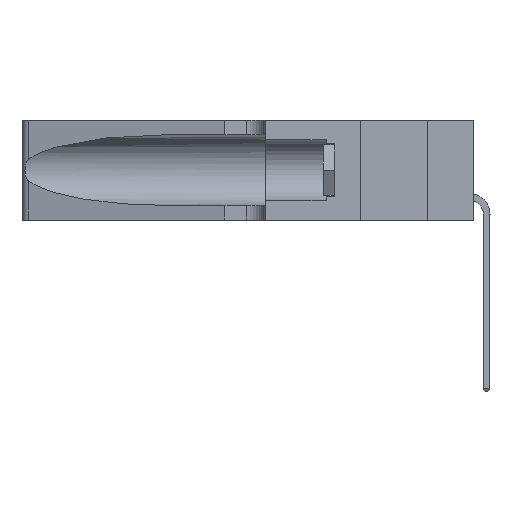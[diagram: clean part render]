
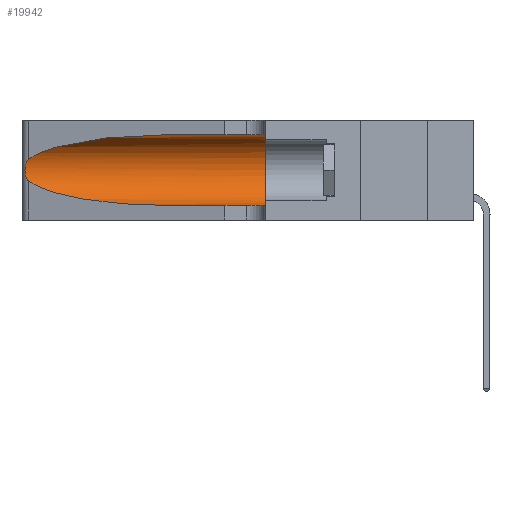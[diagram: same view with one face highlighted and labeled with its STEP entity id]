
A CAD part, left-side view. The second image highlights one B-rep face of the part: STEP entity #19942.
In plain terms, the highlighted cylindrical face has radius 3.308 mm (diameter 6.617 mm), a partial arc.
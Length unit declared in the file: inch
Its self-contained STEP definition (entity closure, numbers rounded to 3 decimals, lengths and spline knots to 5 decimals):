
#207 = ORIENTED_EDGE ( 'NONE', *, *, #4473, .T. ) ;
#224 = CYLINDRICAL_SURFACE ( 'NONE', #10447, 0.13025 ) ;
#479 = CARTESIAN_POINT ( 'NONE',  ( 0.1305, 0.35, 0.185 ) ) ;
#815 = VERTEX_POINT ( 'NONE', #22524 ) ;
#1253 = VERTEX_POINT ( 'NONE', #10271 ) ;
#1884 = ORIENTED_EDGE ( 'NONE', *, *, #13714, .T. ) ;
#2451 = EDGE_CURVE ( 'NONE', #815, #11251, #8190, .T. ) ;
#3369 = B_SPLINE_CURVE_WITH_KNOTS ( 'NONE', 3,
 ( #25205, #7468, #23319, #19471, #9430, #23067, #21374, #25117, #13320, #15282, #7627, #21288, #3598, #9603 ),
 .UNSPECIFIED., .F., .F.,
 ( 4, 2, 2, 2, 2, 2, 4 ),
 ( 0., 0.00027, 0.00053, 0.00107, 0.0016, 0.00187, 0.00214 ),
 .UNSPECIFIED. ) ;
#3598 = CARTESIAN_POINT ( 'NONE',  ( 0.25555, 1.22993, 0.14849 ) ) ;
#4473 = EDGE_CURVE ( 'NONE', #6170, #23893, #11679, .T. ) ;
#5448 = DIRECTION ( 'NONE',  ( 0., -1., 0. ) ) ;
#5451 = CARTESIAN_POINT ( 'NONE',  ( 0.1305, 0.35, 0.05475 ) ) ;
#6170 = VERTEX_POINT ( 'NONE', #17905 ) ;
#6480 =( BOUNDED_CURVE ( )  B_SPLINE_CURVE ( 3, ( #14919, #10932, #22724, #18782 ),
 .UNSPECIFIED., .F., .T. ) 
 B_SPLINE_CURVE_WITH_KNOTS ( ( 4, 4 ),
 ( 3.44316, 4.71239 ),
 .UNSPECIFIED. ) 
 CURVE ( )  GEOMETRIC_REPRESENTATION_ITEM ( )  RATIONAL_B_SPLINE_CURVE ( ( 1., 0.87, 0.87, 1. ) ) 
 REPRESENTATION_ITEM ( '' )  );
#6669 = DIRECTION ( 'NONE',  ( 0., -1., 0. ) ) ;
#6790 = CARTESIAN_POINT ( 'NONE',  ( 0.1305, 0.72297, 0.31525 ) ) ;
#6920 = ORIENTED_EDGE ( 'NONE', *, *, #21639, .T. ) ;
#7079 = ORIENTED_EDGE ( 'NONE', *, *, #13544, .F. ) ;
#7192 = VECTOR ( 'NONE', #5448, 39.37008 ) ;
#7277 = VECTOR ( 'NONE', #6669, 39.37008 ) ;
#7369 = DIRECTION ( 'NONE',  ( 0., -1., 0. ) ) ;
#7468 = CARTESIAN_POINT ( 'NONE',  ( 0.25555, 1.22994, 0.2215 ) ) ;
#7627 = CARTESIAN_POINT ( 'NONE',  ( 0.25789, 1.23486, 0.15765 ) ) ;
#8190 = CIRCLE ( 'NONE', #16425, 0.13025 ) ;
#8674 = CARTESIAN_POINT ( 'NONE',  ( 0.25487, 1.22718, 0.22369 ) ) ;
#9430 = CARTESIAN_POINT ( 'NONE',  ( 0.25854, 1.2359, 0.20912 ) ) ;
#9603 = CARTESIAN_POINT ( 'NONE',  ( 0.25487, 1.22718, 0.14631 ) ) ;
#10034 = CARTESIAN_POINT ( 'NONE',  ( 0.1305, 1.61858, 0.05475 ) ) ;
#10271 = CARTESIAN_POINT ( 'NONE',  ( 0.1305, 0.72297, 0.05475 ) ) ;
#10447 = AXIS2_PLACEMENT_3D ( 'NONE', #16976, #7369, #22961 ) ;
#10672 = FACE_OUTER_BOUND ( 'NONE', #19286, .T. ) ;
#10926 = LINE ( 'NONE', #10034, #7277 ) ;
#10932 = CARTESIAN_POINT ( 'NONE',  ( 0.2373, 1.15595, 0.08982 ) ) ;
#11251 = VERTEX_POINT ( 'NONE', #5451 ) ;
#11390 = ORIENTED_EDGE ( 'NONE', *, *, #2451, .F. ) ;
#11394 = EDGE_CURVE ( 'NONE', #23058, #1253, #6480, .T. ) ;
#11679 =( BOUNDED_CURVE ( )  B_SPLINE_CURVE ( 3, ( #6790, #18476, #22412, #8674 ),
 .UNSPECIFIED., .F., .F. ) 
 B_SPLINE_CURVE_WITH_KNOTS ( ( 4, 4 ),
 ( 1.5708, 2.84003 ),
 .UNSPECIFIED. ) 
 CURVE ( )  GEOMETRIC_REPRESENTATION_ITEM ( )  RATIONAL_B_SPLINE_CURVE ( ( 1., 0.87, 0.87, 1. ) ) 
 REPRESENTATION_ITEM ( '' )  );
#13320 = CARTESIAN_POINT ( 'NONE',  ( 0.26017, 1.23833, 0.17102 ) ) ;
#13544 = EDGE_CURVE ( 'NONE', #6170, #815, #14460, .T. ) ;
#13714 = EDGE_CURVE ( 'NONE', #23893, #23058, #3369, .T. ) ;
#14460 = LINE ( 'NONE', #17147, #7192 ) ;
#14919 = CARTESIAN_POINT ( 'NONE',  ( 0.25487, 1.22718, 0.14631 ) ) ;
#15282 = CARTESIAN_POINT ( 'NONE',  ( 0.25856, 1.23593, 0.16098 ) ) ;
#16425 = AXIS2_PLACEMENT_3D ( 'NONE', #479, #17156, #18959 ) ;
#16835 = ORIENTED_EDGE ( 'NONE', *, *, #11394, .T. ) ;
#16976 = CARTESIAN_POINT ( 'NONE',  ( 0.1305, 1.61858, 0.185 ) ) ;
#17147 = CARTESIAN_POINT ( 'NONE',  ( 0.1305, 1.61858, 0.31525 ) ) ;
#17156 = DIRECTION ( 'NONE',  ( 0., 1., 0. ) ) ;
#17905 = CARTESIAN_POINT ( 'NONE',  ( 0.1305, 0.72297, 0.31525 ) ) ;
#18476 = CARTESIAN_POINT ( 'NONE',  ( 0.18966, 0.96281, 0.31525 ) ) ;
#18782 = CARTESIAN_POINT ( 'NONE',  ( 0.1305, 0.72297, 0.05475 ) ) ;
#18959 = DIRECTION ( 'NONE',  ( 0., 0., 1. ) ) ;
#19286 = EDGE_LOOP ( 'NONE', ( #207, #1884, #16835, #6920, #11390, #7079 ) ) ;
#19471 = CARTESIAN_POINT ( 'NONE',  ( 0.25787, 1.23484, 0.2124 ) ) ;
#19490 = CARTESIAN_POINT ( 'NONE',  ( 0.25487, 1.22718, 0.14631 ) ) ;
#19942 = ADVANCED_FACE ( 'NONE', ( #10672 ), #224, .F. ) ;
#20657 = CARTESIAN_POINT ( 'NONE',  ( 0.25487, 1.22718, 0.22369 ) ) ;
#21288 = CARTESIAN_POINT ( 'NONE',  ( 0.25639, 1.23186, 0.15144 ) ) ;
#21374 = CARTESIAN_POINT ( 'NONE',  ( 0.26075, 1.23896, 0.19203 ) ) ;
#21639 = EDGE_CURVE ( 'NONE', #1253, #11251, #10926, .T. ) ;
#22412 = CARTESIAN_POINT ( 'NONE',  ( 0.2373, 1.15595, 0.28018 ) ) ;
#22524 = CARTESIAN_POINT ( 'NONE',  ( 0.1305, 0.35, 0.31525 ) ) ;
#22724 = CARTESIAN_POINT ( 'NONE',  ( 0.18966, 0.96281, 0.05475 ) ) ;
#22961 = DIRECTION ( 'NONE',  ( 0., 0., -1. ) ) ;
#23058 = VERTEX_POINT ( 'NONE', #19490 ) ;
#23067 = CARTESIAN_POINT ( 'NONE',  ( 0.26018, 1.23835, 0.19895 ) ) ;
#23319 = CARTESIAN_POINT ( 'NONE',  ( 0.25639, 1.23184, 0.21858 ) ) ;
#23893 = VERTEX_POINT ( 'NONE', #20657 ) ;
#25117 = CARTESIAN_POINT ( 'NONE',  ( 0.26075, 1.23896, 0.178 ) ) ;
#25205 = CARTESIAN_POINT ( 'NONE',  ( 0.25487, 1.22718, 0.22369 ) ) ;
